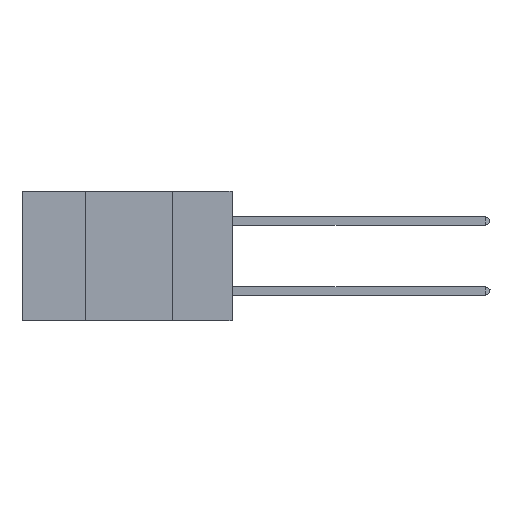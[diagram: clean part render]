
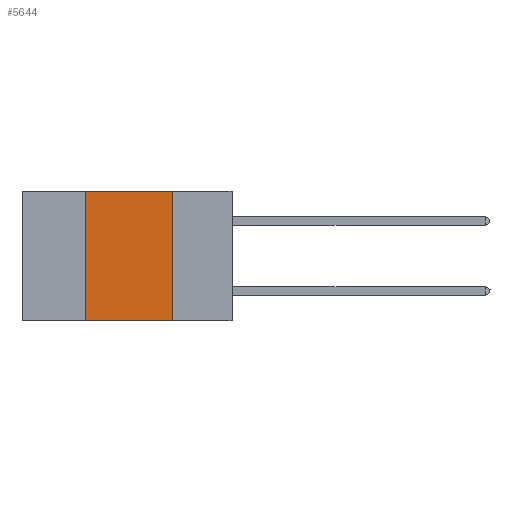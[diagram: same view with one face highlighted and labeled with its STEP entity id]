
A CAD part, left-side view. The second image highlights one B-rep face of the part: STEP entity #5644.
In plain terms, the highlighted planar face has unit normal (-1, 0, 0).
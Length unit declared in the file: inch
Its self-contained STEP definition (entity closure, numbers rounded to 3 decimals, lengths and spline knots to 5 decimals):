
#872 = CARTESIAN_POINT ( 'NONE',  ( 0., 0.17, 0. ) ) ;
#1355 = DIRECTION ( 'NONE',  ( 0., -1., 0. ) ) ;
#1629 = ORIENTED_EDGE ( 'NONE', *, *, #3878, .F. ) ;
#1704 = PLANE ( 'NONE',  #15660 ) ;
#2681 = DIRECTION ( 'NONE',  ( 0., -1., 0. ) ) ;
#2835 = CARTESIAN_POINT ( 'NONE',  ( 0., 0.17, -0.37 ) ) ;
#3216 = VERTEX_POINT ( 'NONE', #2835 ) ;
#3271 = VERTEX_POINT ( 'NONE', #11500 ) ;
#3878 = EDGE_CURVE ( 'NONE', #11883, #3271, #16159, .T. ) ;
#4108 = EDGE_CURVE ( 'NONE', #7559, #3216, #8767, .T. ) ;
#5537 = FACE_OUTER_BOUND ( 'NONE', #7975, .T. ) ;
#5644 = ADVANCED_FACE ( 'NONE', ( #5537 ), #1704, .F. ) ;
#5892 = LINE ( 'NONE', #10980, #16703 ) ;
#7458 = DIRECTION ( 'NONE',  ( 0., 0., -1. ) ) ;
#7559 = VERTEX_POINT ( 'NONE', #15380 ) ;
#7838 = ORIENTED_EDGE ( 'NONE', *, *, #8687, .T. ) ;
#7975 = EDGE_LOOP ( 'NONE', ( #14455, #10992, #1629, #7838 ) ) ;
#8687 = EDGE_CURVE ( 'NONE', #11883, #3216, #5892, .T. ) ;
#8767 = LINE ( 'NONE', #872, #17628 ) ;
#8777 = DIRECTION ( 'NONE',  ( 1., 0., 0. ) ) ;
#9612 = DIRECTION ( 'NONE',  ( 0., 0., 1. ) ) ;
#9895 = CARTESIAN_POINT ( 'NONE',  ( 0., 0.6, 0. ) ) ;
#10357 = LINE ( 'NONE', #9895, #12726 ) ;
#10472 = DIRECTION ( 'NONE',  ( 0., 0., -1. ) ) ;
#10751 = VECTOR ( 'NONE', #9612, 39.37008 ) ;
#10836 = EDGE_CURVE ( 'NONE', #3271, #7559, #10357, .T. ) ;
#10980 = CARTESIAN_POINT ( 'NONE',  ( 0., 0.6, -0.37 ) ) ;
#10992 = ORIENTED_EDGE ( 'NONE', *, *, #10836, .F. ) ;
#11500 = CARTESIAN_POINT ( 'NONE',  ( 0., 0.42, 0. ) ) ;
#11883 = VERTEX_POINT ( 'NONE', #14867 ) ;
#12726 = VECTOR ( 'NONE', #2681, 39.37008 ) ;
#12891 = CARTESIAN_POINT ( 'NONE',  ( 0., 0.6, 0. ) ) ;
#14455 = ORIENTED_EDGE ( 'NONE', *, *, #4108, .F. ) ;
#14867 = CARTESIAN_POINT ( 'NONE',  ( 0., 0.42, -0.37 ) ) ;
#15036 = CARTESIAN_POINT ( 'NONE',  ( 0., 0.42, 0. ) ) ;
#15380 = CARTESIAN_POINT ( 'NONE',  ( 0., 0.17, 0. ) ) ;
#15660 = AXIS2_PLACEMENT_3D ( 'NONE', #12891, #8777, #10472 ) ;
#16159 = LINE ( 'NONE', #15036, #10751 ) ;
#16703 = VECTOR ( 'NONE', #1355, 39.37008 ) ;
#17628 = VECTOR ( 'NONE', #7458, 39.37008 ) ;
